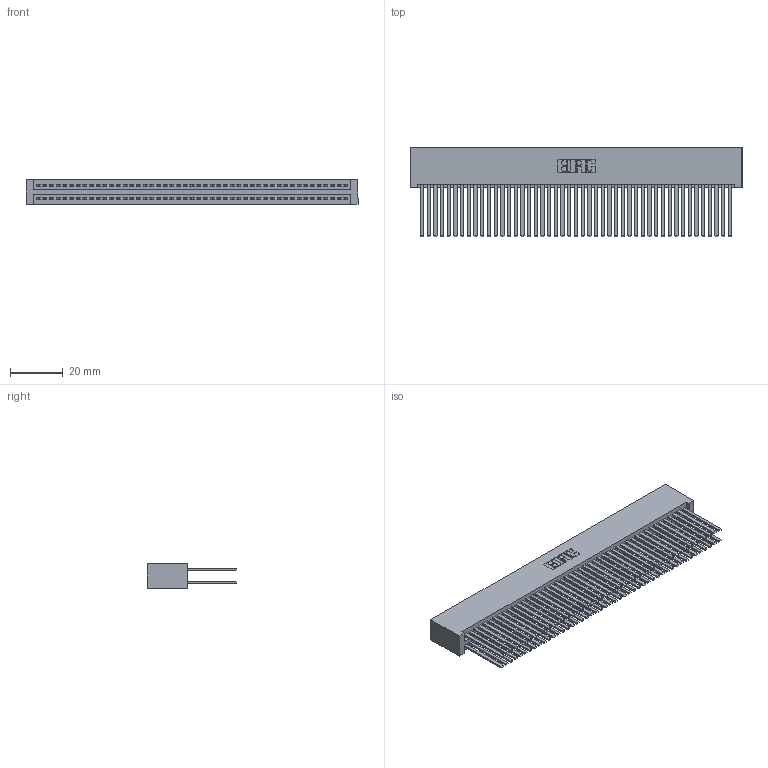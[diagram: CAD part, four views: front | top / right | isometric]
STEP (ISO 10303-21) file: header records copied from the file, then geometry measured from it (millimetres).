
FILE_DESCRIPTION (( 'STEP AP203' ), '1' );
FILE_NAME ('395-094-544-201.STEP', '2018-11-29T12:51:49', ( '' ), ( '' ), 'SwSTEP 2.0', 'SolidWorks 2016', '' );
FILE_SCHEMA (( 'CONFIG_CONTROL_DESIGN' ));
Length unit declared in the file: inch
Products named in the file (3): 345 Part_No Mounting Lugs; 345-292-001_345-293-144; 395-094-544-201
Assembly tree (95 placements, depth 2):
  395-094-544-201
    345 Part_No Mounting Lugs
    345-292-001_345-293-144  x94
Bounding box: 125.98 x 33.96 x 9.4 mm (x, y, z)
Volume: 14218.2 mm3; surface area: 25279.1 mm2
Topology: 95 solids, 95 shells, 4254 faces, 12631 edges, 8294 vertices
Faces by surface type: plane 2802, cylinder 1452
Entity records: 35743 total; most frequent: CARTESIAN_POINT 5984, ORIENTED_EDGE 5918, DIRECTION 5263, EDGE_CURVE 2959, LINE 2651, VECTOR 2651, VERTEX_POINT 1970, AXIS2_PLACEMENT_3D 1306
